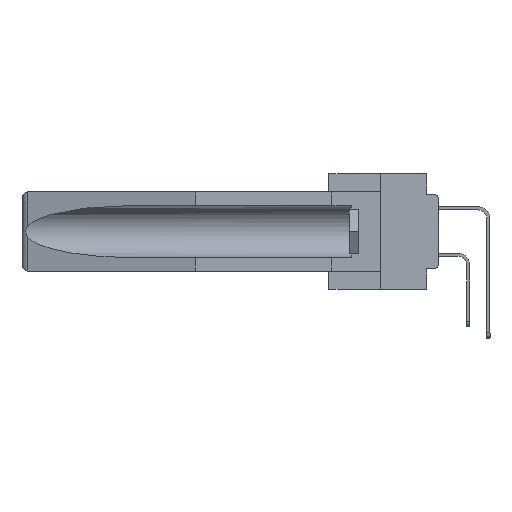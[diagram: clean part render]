
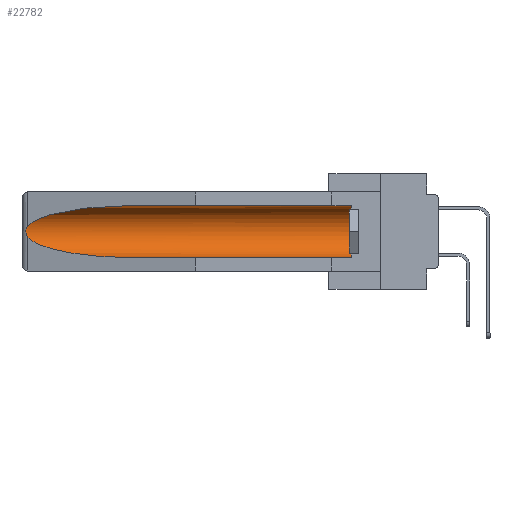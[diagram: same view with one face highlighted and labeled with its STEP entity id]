
A CAD part, left-side view. The second image highlights one B-rep face of the part: STEP entity #22782.
In plain terms, the highlighted cylindrical face has radius 2.857 mm (diameter 5.715 mm), a partial arc.
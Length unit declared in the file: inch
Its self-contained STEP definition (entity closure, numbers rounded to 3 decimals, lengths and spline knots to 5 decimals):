
#566 = CARTESIAN_POINT ( 'NONE',  ( 0.2675, 1.53308, -0.16763 ) ) ;
#726 = CARTESIAN_POINT ( 'NONE',  ( 0.26537, 1.52718, -0.14972 ) ) ;
#1505 = AXIS2_PLACEMENT_3D ( 'NONE', #30239, #8811, #27806 ) ;
#1537 = EDGE_CURVE ( 'NONE', #19161, #19504, #31961, .T. ) ;
#3171 = CARTESIAN_POINT ( 'NONE',  ( 0.26537, 1.52718, -0.19328 ) ) ;
#3334 = CARTESIAN_POINT ( 'NONE',  ( 0.26597, 1.5296, -0.19026 ) ) ;
#3521 = LINE ( 'NONE', #6129, #6518 ) ;
#3946 = VERTEX_POINT ( 'NONE', #30540 ) ;
#4790 = CARTESIAN_POINT ( 'NONE',  ( 0.26537, 1.52718, -0.19328 ) ) ;
#4965 = CARTESIAN_POINT ( 'NONE',  ( 0.21114, 1.30732, -0.284 ) ) ;
#6129 = CARTESIAN_POINT ( 'NONE',  ( 0.155, -0.30754, -0.284 ) ) ;
#6518 = VECTOR ( 'NONE', #13609, 39.37008 ) ;
#6536 = CARTESIAN_POINT ( 'NONE',  ( 0.155, -0.30754, -0.1715 ) ) ;
#7309 = CARTESIAN_POINT ( 'NONE',  ( 0.155, 1.07973, -0.059 ) ) ;
#8149 = DIRECTION ( 'NONE',  ( 0., 1., 0. ) ) ;
#8321 = CARTESIAN_POINT ( 'NONE',  ( 0.155, -0.30754, -0.059 ) ) ;
#8698 = CIRCLE ( 'NONE', #1505, 0.1125 ) ;
#8709 = CARTESIAN_POINT ( 'NONE',  ( 0.2673, 1.5327, -0.16383 ) ) ;
#8811 = DIRECTION ( 'NONE',  ( 0., -1., 0. ) ) ;
#10353 =( BOUNDED_CURVE ( )  B_SPLINE_CURVE ( 3, ( #4790, #13470, #4965, #31431 ),
 .UNSPECIFIED., .F., .F. ) 
 B_SPLINE_CURVE_WITH_KNOTS ( ( 4, 4 ),
 ( 0.1948, 1.5708 ),
 .UNSPECIFIED. ) 
 CURVE ( )  GEOMETRIC_REPRESENTATION_ITEM ( )  RATIONAL_B_SPLINE_CURVE ( ( 1., 0.848, 0.848, 1. ) ) 
 REPRESENTATION_ITEM ( '' )  );
#10597 = VECTOR ( 'NONE', #8149, 39.37008 ) ;
#10997 = VERTEX_POINT ( 'NONE', #7309 ) ;
#11423 = FACE_OUTER_BOUND ( 'NONE', #33119, .T. ) ;
#11991 = VERTEX_POINT ( 'NONE', #21835 ) ;
#13470 = CARTESIAN_POINT ( 'NONE',  ( 0.25451, 1.48313, -0.24835 ) ) ;
#13529 = EDGE_CURVE ( 'NONE', #16068, #10997, #31512, .T. ) ;
#13609 = DIRECTION ( 'NONE',  ( 0., 1., 0. ) ) ;
#15669 = EDGE_CURVE ( 'NONE', #19504, #3946, #10353, .T. ) ;
#16051 = CARTESIAN_POINT ( 'NONE',  ( 0.26537, 1.52718, -0.14972 ) ) ;
#16068 = VERTEX_POINT ( 'NONE', #30541 ) ;
#16281 = ORIENTED_EDGE ( 'NONE', *, *, #15669, .T. ) ;
#16403 = CARTESIAN_POINT ( 'NONE',  ( 0.26655, 1.53094, -0.18657 ) ) ;
#16567 = CARTESIAN_POINT ( 'NONE',  ( 0.26537, 1.52718, -0.14972 ) ) ;
#16748 = CARTESIAN_POINT ( 'NONE',  ( 0.2675, 1.53308, -0.17534 ) ) ;
#16892 = CARTESIAN_POINT ( 'NONE',  ( 0.21114, 1.30732, -0.059 ) ) ;
#17059 = ORIENTED_EDGE ( 'NONE', *, *, #24952, .F. ) ;
#18461 = ORIENTED_EDGE ( 'NONE', *, *, #28994, .T. ) ;
#19161 = VERTEX_POINT ( 'NONE', #16051 ) ;
#19504 = VERTEX_POINT ( 'NONE', #31639 ) ;
#21473 = CARTESIAN_POINT ( 'NONE',  ( 0.26654, 1.53092, -0.15636 ) ) ;
#21656 = ORIENTED_EDGE ( 'NONE', *, *, #13529, .T. ) ;
#21835 = CARTESIAN_POINT ( 'NONE',  ( 0.155, 0.126, -0.284 ) ) ;
#22087 = CYLINDRICAL_SURFACE ( 'NONE', #26429, 0.1125 ) ;
#22782 = ADVANCED_FACE ( 'NONE', ( #11423 ), #22087, .F. ) ;
#24097 = EDGE_CURVE ( 'NONE', #11991, #16068, #8698, .T. ) ;
#24551 = CARTESIAN_POINT ( 'NONE',  ( 0.155, 1.07973, -0.059 ) ) ;
#24952 = EDGE_CURVE ( 'NONE', #11991, #3946, #3521, .T. ) ;
#24996 = DIRECTION ( 'NONE',  ( 0., 1., 0. ) ) ;
#26429 = AXIS2_PLACEMENT_3D ( 'NONE', #6536, #24996, #32680 ) ;
#26957 = ORIENTED_EDGE ( 'NONE', *, *, #1537, .T. ) ;
#27059 =( BOUNDED_CURVE ( )  B_SPLINE_CURVE ( 3, ( #24551, #16892, #27514, #16567 ),
 .UNSPECIFIED., .F., .F. ) 
 B_SPLINE_CURVE_WITH_KNOTS ( ( 4, 4 ),
 ( 4.71239, 6.08839 ),
 .UNSPECIFIED. ) 
 CURVE ( )  GEOMETRIC_REPRESENTATION_ITEM ( )  RATIONAL_B_SPLINE_CURVE ( ( 1., 0.848, 0.848, 1. ) ) 
 REPRESENTATION_ITEM ( '' )  );
#27360 = CARTESIAN_POINT ( 'NONE',  ( 0.2673, 1.53269, -0.17917 ) ) ;
#27514 = CARTESIAN_POINT ( 'NONE',  ( 0.25451, 1.48313, -0.09465 ) ) ;
#27806 = DIRECTION ( 'NONE',  ( 0., 0., 1. ) ) ;
#28994 = EDGE_CURVE ( 'NONE', #10997, #19161, #27059, .T. ) ;
#29494 = ORIENTED_EDGE ( 'NONE', *, *, #24097, .T. ) ;
#29800 = CARTESIAN_POINT ( 'NONE',  ( 0.26597, 1.52961, -0.15275 ) ) ;
#30239 = CARTESIAN_POINT ( 'NONE',  ( 0.155, 0.126, -0.1715 ) ) ;
#30540 = CARTESIAN_POINT ( 'NONE',  ( 0.155, 1.07973, -0.284 ) ) ;
#30541 = CARTESIAN_POINT ( 'NONE',  ( 0.155, 0.126, -0.059 ) ) ;
#31431 = CARTESIAN_POINT ( 'NONE',  ( 0.155, 1.07973, -0.284 ) ) ;
#31512 = LINE ( 'NONE', #8321, #10597 ) ;
#31639 = CARTESIAN_POINT ( 'NONE',  ( 0.26537, 1.52718, -0.19328 ) ) ;
#31961 = B_SPLINE_CURVE_WITH_KNOTS ( 'NONE', 3,
 ( #726, #29800, #21473, #8709, #566, #16748, #27360, #16403, #3334, #3171 ),
 .UNSPECIFIED., .F., .F.,
 ( 4, 2, 2, 2, 4 ),
 ( 0., 0.00029, 0.00058, 0.00087, 0.00117 ),
 .UNSPECIFIED. ) ;
#32680 = DIRECTION ( 'NONE',  ( 0., 0., 1. ) ) ;
#33119 = EDGE_LOOP ( 'NONE', ( #18461, #26957, #16281, #17059, #29494, #21656 ) ) ;
